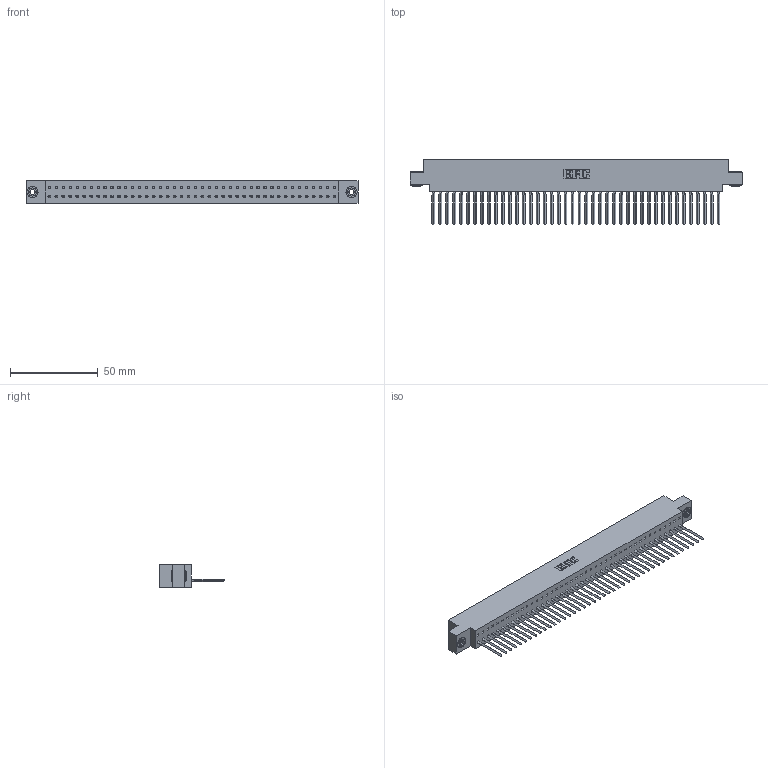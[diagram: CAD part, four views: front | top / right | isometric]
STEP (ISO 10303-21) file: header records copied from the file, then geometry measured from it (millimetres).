
FILE_DESCRIPTION (( 'STEP AP203' ), '1' );
FILE_NAME ('317-042-541-603.STEP', '2020-02-28T01:12:29', ( '' ), ( '' ), 'SwSTEP 2.0', 'SolidWorks 2016', '' );
FILE_SCHEMA (( 'CONFIG_CONTROL_DESIGN' ));
Length unit declared in the file: inch
Products named in the file (4): 345-250-002_345-250-002-102; 317 Part_.156 Dia - TH; 317-042-541-603; 317-290-002_541
Assembly tree (45 placements, depth 2):
  317-042-541-603
    317 Part_.156 Dia - TH
    317-290-002_541  x42
    345-250-002_345-250-002-102  x2
Bounding box: 189.13 x 37.34 x 12.7 mm (x, y, z)
Volume: 30689.7 mm3; surface area: 43581.2 mm2
Topology: 45 solids, 45 shells, 6524 faces, 18579 edges, 12074 vertices
Faces by surface type: plane 5276, cylinder 1072, bspline 168, cone 8
Entity records: 61565 total; most frequent: CARTESIAN_POINT 11554, ORIENTED_EDGE 10842, DIRECTION 8947, EDGE_CURVE 5421, LINE 5033, VECTOR 5033, VERTEX_POINT 3604, AXIS2_PLACEMENT_3D 1957
